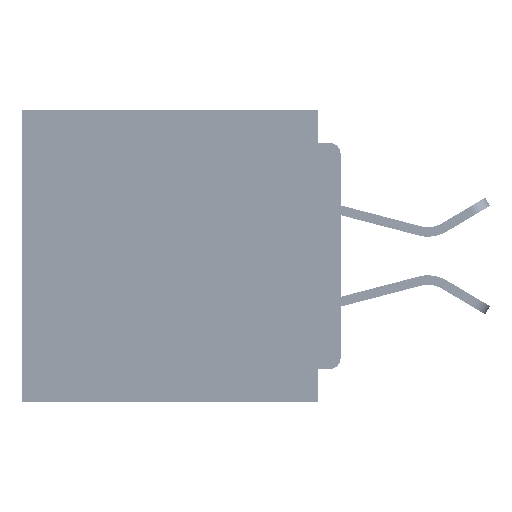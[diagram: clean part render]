
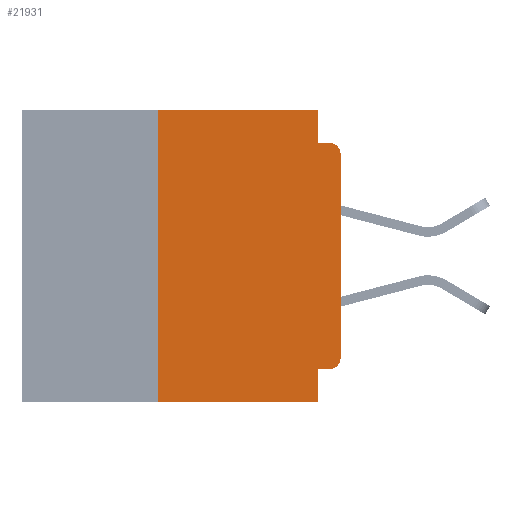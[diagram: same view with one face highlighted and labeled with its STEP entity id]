
A CAD part, left-side view. The second image highlights one B-rep face of the part: STEP entity #21931.
In plain terms, the highlighted planar face has unit normal (-1, 0, 0).
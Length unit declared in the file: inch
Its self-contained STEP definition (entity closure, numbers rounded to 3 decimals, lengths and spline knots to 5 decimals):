
#351 = ORIENTED_EDGE ( 'NONE', *, *, #19806, .F. ) ;
#1485 = CARTESIAN_POINT ( 'NONE',  ( 0., 0.015, -0.045 ) ) ;
#1595 = EDGE_LOOP ( 'NONE', ( #16623, #17768, #28601, #32982, #7359, #23926, #43899, #351, #32260, #24725 ) ) ;
#3118 = CARTESIAN_POINT ( 'NONE',  ( 0., 0.25, -0.4 ) ) ;
#3488 = CARTESIAN_POINT ( 'NONE',  ( 0., 0.015, -0.355 ) ) ;
#3757 = EDGE_CURVE ( 'NONE', #28127, #37133, #9433, .T. ) ;
#3954 = CARTESIAN_POINT ( 'NONE',  ( 0., 0.25, 0. ) ) ;
#4958 = CARTESIAN_POINT ( 'NONE',  ( 0., 0., -0.355 ) ) ;
#5532 = DIRECTION ( 'NONE',  ( 0., 0., 1. ) ) ;
#5569 = EDGE_CURVE ( 'NONE', #7404, #7304, #53891, .T. ) ;
#6056 = LINE ( 'NONE', #4958, #49526 ) ;
#6158 = VERTEX_POINT ( 'NONE', #3954 ) ;
#7304 = VERTEX_POINT ( 'NONE', #1485 ) ;
#7359 = ORIENTED_EDGE ( 'NONE', *, *, #31038, .F. ) ;
#7404 = VERTEX_POINT ( 'NONE', #15234 ) ;
#9433 = CIRCLE ( 'NONE', #36379, 0.015 ) ;
#9536 = CARTESIAN_POINT ( 'NONE',  ( 0., 0.437, 0. ) ) ;
#9798 = AXIS2_PLACEMENT_3D ( 'NONE', #13954, #43268, #18220 ) ;
#11809 = VECTOR ( 'NONE', #5532, 39.37008 ) ;
#13954 = CARTESIAN_POINT ( 'NONE',  ( 0., 0.015, -0.06 ) ) ;
#15234 = CARTESIAN_POINT ( 'NONE',  ( 0., 0.031, -0.045 ) ) ;
#15861 = VECTOR ( 'NONE', #41357, 39.37008 ) ;
#16623 = ORIENTED_EDGE ( 'NONE', *, *, #53509, .T. ) ;
#17504 = VECTOR ( 'NONE', #39760, 39.37008 ) ;
#17768 = ORIENTED_EDGE ( 'NONE', *, *, #20937, .T. ) ;
#18220 = DIRECTION ( 'NONE',  ( 0., 0., -1. ) ) ;
#18851 = DIRECTION ( 'NONE',  ( 1., 0., 0. ) ) ;
#19317 = CIRCLE ( 'NONE', #9798, 0.015 ) ;
#19806 = EDGE_CURVE ( 'NONE', #20505, #30699, #53469, .T. ) ;
#20505 = VERTEX_POINT ( 'NONE', #53008 ) ;
#20937 = EDGE_CURVE ( 'NONE', #41430, #7304, #19317, .T. ) ;
#21548 = DIRECTION ( 'NONE',  ( -1., 0., 0. ) ) ;
#21931 = ADVANCED_FACE ( 'NONE', ( #43392 ), #43893, .F. ) ;
#22486 = CARTESIAN_POINT ( 'NONE',  ( 0., 0.25, -0.4 ) ) ;
#23030 = LINE ( 'NONE', #22486, #11809 ) ;
#23926 = ORIENTED_EDGE ( 'NONE', *, *, #47827, .F. ) ;
#24031 = CARTESIAN_POINT ( 'NONE',  ( 0., 0.031, 0. ) ) ;
#24725 = ORIENTED_EDGE ( 'NONE', *, *, #3757, .T. ) ;
#26571 = DIRECTION ( 'NONE',  ( 0., -1., 0. ) ) ;
#27731 = VECTOR ( 'NONE', #45657, 39.37008 ) ;
#28076 = VERTEX_POINT ( 'NONE', #3118 ) ;
#28127 = VERTEX_POINT ( 'NONE', #3488 ) ;
#28601 = ORIENTED_EDGE ( 'NONE', *, *, #5569, .F. ) ;
#29297 = AXIS2_PLACEMENT_3D ( 'NONE', #39708, #18851, #48106 ) ;
#29642 = LINE ( 'NONE', #9536, #50545 ) ;
#30699 = VERTEX_POINT ( 'NONE', #40999 ) ;
#30958 = VECTOR ( 'NONE', #49235, 39.37008 ) ;
#31038 = EDGE_CURVE ( 'NONE', #6158, #46101, #29642, .T. ) ;
#32260 = ORIENTED_EDGE ( 'NONE', *, *, #34982, .F. ) ;
#32284 = LINE ( 'NONE', #24031, #30958 ) ;
#32982 = ORIENTED_EDGE ( 'NONE', *, *, #53434, .F. ) ;
#33869 = EDGE_CURVE ( 'NONE', #28076, #30699, #50862, .T. ) ;
#34982 = EDGE_CURVE ( 'NONE', #28127, #20505, #6056, .T. ) ;
#35583 = CARTESIAN_POINT ( 'NONE',  ( 0., 0.437, -0.4 ) ) ;
#36379 = AXIS2_PLACEMENT_3D ( 'NONE', #46587, #21548, #50785 ) ;
#37133 = VERTEX_POINT ( 'NONE', #51113 ) ;
#38422 = VECTOR ( 'NONE', #48504, 39.37008 ) ;
#39708 = CARTESIAN_POINT ( 'NONE',  ( 0., 0.437, 0. ) ) ;
#39760 = DIRECTION ( 'NONE',  ( 0., -1., 0. ) ) ;
#40999 = CARTESIAN_POINT ( 'NONE',  ( 0., 0.031, -0.4 ) ) ;
#41357 = DIRECTION ( 'NONE',  ( 0., 0., 1. ) ) ;
#41430 = VERTEX_POINT ( 'NONE', #43914 ) ;
#42920 = DIRECTION ( 'NONE',  ( 0., 1., 0. ) ) ;
#43268 = DIRECTION ( 'NONE',  ( -1., 0., 0. ) ) ;
#43392 = FACE_OUTER_BOUND ( 'NONE', #1595, .T. ) ;
#43893 = PLANE ( 'NONE',  #29297 ) ;
#43899 = ORIENTED_EDGE ( 'NONE', *, *, #33869, .T. ) ;
#43914 = CARTESIAN_POINT ( 'NONE',  ( 0., 0., -0.06 ) ) ;
#44312 = CARTESIAN_POINT ( 'NONE',  ( 0., 0.031, -0.4 ) ) ;
#45657 = DIRECTION ( 'NONE',  ( 0., -1., 0. ) ) ;
#46101 = VERTEX_POINT ( 'NONE', #46430 ) ;
#46430 = CARTESIAN_POINT ( 'NONE',  ( 0., 0.031, 0. ) ) ;
#46587 = CARTESIAN_POINT ( 'NONE',  ( 0., 0.015, -0.34 ) ) ;
#47827 = EDGE_CURVE ( 'NONE', #28076, #6158, #23030, .T. ) ;
#48106 = DIRECTION ( 'NONE',  ( 0., 0., -1. ) ) ;
#48504 = DIRECTION ( 'NONE',  ( 0., 0., -1. ) ) ;
#49235 = DIRECTION ( 'NONE',  ( 0., 0., -1. ) ) ;
#49247 = LINE ( 'NONE', #49595, #15861 ) ;
#49526 = VECTOR ( 'NONE', #42920, 39.37008 ) ;
#49595 = CARTESIAN_POINT ( 'NONE',  ( 0., 0., 0. ) ) ;
#49877 = CARTESIAN_POINT ( 'NONE',  ( 0., 0., -0.045 ) ) ;
#50545 = VECTOR ( 'NONE', #26571, 39.37008 ) ;
#50785 = DIRECTION ( 'NONE',  ( 0., 0., -1. ) ) ;
#50862 = LINE ( 'NONE', #35583, #17504 ) ;
#51113 = CARTESIAN_POINT ( 'NONE',  ( 0., 0., -0.34 ) ) ;
#53008 = CARTESIAN_POINT ( 'NONE',  ( 0., 0.031, -0.355 ) ) ;
#53434 = EDGE_CURVE ( 'NONE', #46101, #7404, #32284, .T. ) ;
#53469 = LINE ( 'NONE', #44312, #38422 ) ;
#53509 = EDGE_CURVE ( 'NONE', #37133, #41430, #49247, .T. ) ;
#53891 = LINE ( 'NONE', #49877, #27731 ) ;
